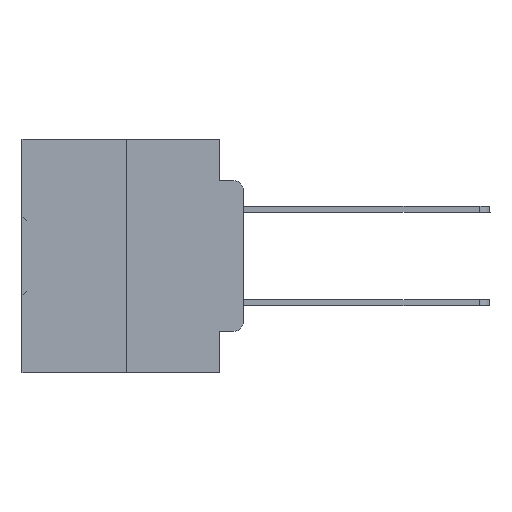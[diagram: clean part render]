
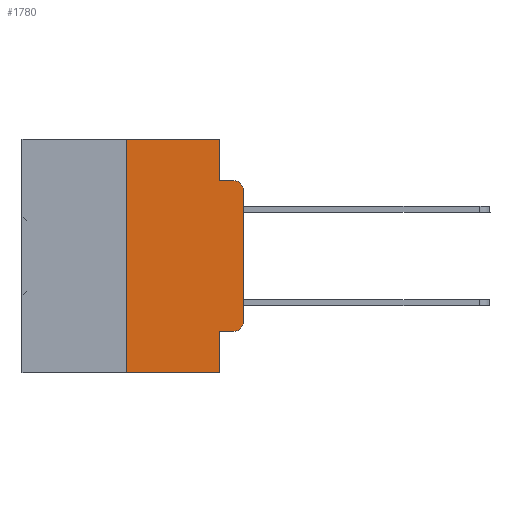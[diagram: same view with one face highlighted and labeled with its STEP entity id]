
A CAD part, left-side view. The second image highlights one B-rep face of the part: STEP entity #1780.
In plain terms, the highlighted planar face has unit normal (-1, 0, 0).
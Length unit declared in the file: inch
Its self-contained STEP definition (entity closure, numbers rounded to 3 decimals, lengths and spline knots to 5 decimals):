
#184 = ORIENTED_EDGE ( 'NONE', *, *, #28076, .T. ) ;
#339 = DIRECTION ( 'NONE',  ( -1., 0., 0. ) ) ;
#488 = LINE ( 'NONE', #30075, #31539 ) ;
#667 = DIRECTION ( 'NONE',  ( 0., -1., 0. ) ) ;
#1204 = CIRCLE ( 'NONE', #9389, 0.02 ) ;
#1375 = CARTESIAN_POINT ( 'NONE',  ( 0., 0.02, -0.1085 ) ) ;
#1562 = ORIENTED_EDGE ( 'NONE', *, *, #8006, .T. ) ;
#1780 = ADVANCED_FACE ( 'NONE', ( #26028 ), #14416, .F. ) ;
#1823 = CARTESIAN_POINT ( 'NONE',  ( 0., 0.051, 0. ) ) ;
#2549 = AXIS2_PLACEMENT_3D ( 'NONE', #1375, #21821, #4304 ) ;
#2571 = VECTOR ( 'NONE', #5016, 39.37008 ) ;
#3223 = EDGE_LOOP ( 'NONE', ( #20301, #1562, #24870, #10236, #19879, #22594, #184, #31233, #27148, #28967 ) ) ;
#3599 = CARTESIAN_POINT ( 'NONE',  ( 0., 0.051, 0. ) ) ;
#3652 = DIRECTION ( 'NONE',  ( 0., -1., 0. ) ) ;
#3897 = CARTESIAN_POINT ( 'NONE',  ( 0., 0.02, -0.0885 ) ) ;
#4127 = EDGE_CURVE ( 'NONE', #21525, #31232, #7282, .T. ) ;
#4304 = DIRECTION ( 'NONE',  ( 0., 0., -1. ) ) ;
#4619 = CARTESIAN_POINT ( 'NONE',  ( 0., 0.25, 0. ) ) ;
#5016 = DIRECTION ( 'NONE',  ( 0., -1., 0. ) ) ;
#5712 = VERTEX_POINT ( 'NONE', #8740 ) ;
#6056 = EDGE_CURVE ( 'NONE', #31232, #13509, #18146, .T. ) ;
#6818 = LINE ( 'NONE', #22904, #36858 ) ;
#6942 = DIRECTION ( 'NONE',  ( 1., 0., 0. ) ) ;
#7282 = LINE ( 'NONE', #3599, #21940 ) ;
#7541 = CARTESIAN_POINT ( 'NONE',  ( 0., 0.051, 0. ) ) ;
#7807 = CARTESIAN_POINT ( 'NONE',  ( 0., 0.051, -0.0885 ) ) ;
#8006 = EDGE_CURVE ( 'NONE', #28084, #13509, #13012, .T. ) ;
#8740 = CARTESIAN_POINT ( 'NONE',  ( 0., 0.051, -0.4115 ) ) ;
#8937 = VERTEX_POINT ( 'NONE', #34529 ) ;
#9389 = AXIS2_PLACEMENT_3D ( 'NONE', #17890, #339, #20785 ) ;
#10236 = ORIENTED_EDGE ( 'NONE', *, *, #4127, .F. ) ;
#10622 = VERTEX_POINT ( 'NONE', #4619 ) ;
#10963 = DIRECTION ( 'NONE',  ( 0., -1., 0. ) ) ;
#10972 = VECTOR ( 'NONE', #667, 39.37008 ) ;
#12506 = DIRECTION ( 'NONE',  ( 0., 0., 1. ) ) ;
#13012 = CIRCLE ( 'NONE', #2549, 0.02 ) ;
#13450 = DIRECTION ( 'NONE',  ( 0., 0., -1. ) ) ;
#13509 = VERTEX_POINT ( 'NONE', #3897 ) ;
#14416 = PLANE ( 'NONE',  #29544 ) ;
#15369 = CARTESIAN_POINT ( 'NONE',  ( 0., 0., -0.1085 ) ) ;
#15442 = EDGE_CURVE ( 'NONE', #10622, #21525, #24376, .T. ) ;
#16745 = DIRECTION ( 'NONE',  ( 0., 0., -1. ) ) ;
#16824 = VERTEX_POINT ( 'NONE', #33489 ) ;
#17862 = EDGE_CURVE ( 'NONE', #16824, #28084, #488, .T. ) ;
#17890 = CARTESIAN_POINT ( 'NONE',  ( 0., 0.02, -0.3915 ) ) ;
#18146 = LINE ( 'NONE', #7807, #2571 ) ;
#18437 = LINE ( 'NONE', #1823, #20250 ) ;
#19879 = ORIENTED_EDGE ( 'NONE', *, *, #15442, .F. ) ;
#19896 = CARTESIAN_POINT ( 'NONE',  ( 0., 0.051, -0.5 ) ) ;
#20250 = VECTOR ( 'NONE', #13450, 39.37008 ) ;
#20301 = ORIENTED_EDGE ( 'NONE', *, *, #17862, .T. ) ;
#20521 = EDGE_CURVE ( 'NONE', #26332, #16824, #1204, .T. ) ;
#20785 = DIRECTION ( 'NONE',  ( 0., 0., -1. ) ) ;
#21156 = CARTESIAN_POINT ( 'NONE',  ( 0., 0.473, 0. ) ) ;
#21525 = VERTEX_POINT ( 'NONE', #7541 ) ;
#21821 = DIRECTION ( 'NONE',  ( -1., 0., 0. ) ) ;
#21940 = VECTOR ( 'NONE', #24052, 39.37008 ) ;
#22212 = LINE ( 'NONE', #37016, #30849 ) ;
#22529 = VECTOR ( 'NONE', #3652, 39.37008 ) ;
#22594 = ORIENTED_EDGE ( 'NONE', *, *, #34113, .F. ) ;
#22904 = CARTESIAN_POINT ( 'NONE',  ( 0., 0.25, 0. ) ) ;
#24052 = DIRECTION ( 'NONE',  ( 0., 0., -1. ) ) ;
#24376 = LINE ( 'NONE', #21156, #22529 ) ;
#24422 = CARTESIAN_POINT ( 'NONE',  ( 0., 0.02, -0.4115 ) ) ;
#24870 = ORIENTED_EDGE ( 'NONE', *, *, #6056, .F. ) ;
#26028 = FACE_OUTER_BOUND ( 'NONE', #3223, .T. ) ;
#26332 = VERTEX_POINT ( 'NONE', #24422 ) ;
#26478 = LINE ( 'NONE', #29753, #10972 ) ;
#27148 = ORIENTED_EDGE ( 'NONE', *, *, #30275, .T. ) ;
#27285 = VERTEX_POINT ( 'NONE', #19896 ) ;
#27552 = CARTESIAN_POINT ( 'NONE',  ( 0., 0.473, 0. ) ) ;
#28076 = EDGE_CURVE ( 'NONE', #8937, #27285, #26478, .T. ) ;
#28084 = VERTEX_POINT ( 'NONE', #15369 ) ;
#28967 = ORIENTED_EDGE ( 'NONE', *, *, #20521, .T. ) ;
#29544 = AXIS2_PLACEMENT_3D ( 'NONE', #27552, #6942, #16745 ) ;
#29753 = CARTESIAN_POINT ( 'NONE',  ( 0., 0.473, -0.5 ) ) ;
#30075 = CARTESIAN_POINT ( 'NONE',  ( 0., 0., 0. ) ) ;
#30275 = EDGE_CURVE ( 'NONE', #5712, #26332, #22212, .T. ) ;
#30849 = VECTOR ( 'NONE', #10963, 39.37008 ) ;
#31232 = VERTEX_POINT ( 'NONE', #35562 ) ;
#31233 = ORIENTED_EDGE ( 'NONE', *, *, #32190, .F. ) ;
#31539 = VECTOR ( 'NONE', #12506, 39.37008 ) ;
#31664 = DIRECTION ( 'NONE',  ( 0., 0., 1. ) ) ;
#32190 = EDGE_CURVE ( 'NONE', #5712, #27285, #18437, .T. ) ;
#33489 = CARTESIAN_POINT ( 'NONE',  ( 0., 0., -0.3915 ) ) ;
#34113 = EDGE_CURVE ( 'NONE', #8937, #10622, #6818, .T. ) ;
#34529 = CARTESIAN_POINT ( 'NONE',  ( 0., 0.25, -0.5 ) ) ;
#35562 = CARTESIAN_POINT ( 'NONE',  ( 0., 0.051, -0.0885 ) ) ;
#36858 = VECTOR ( 'NONE', #31664, 39.37008 ) ;
#37016 = CARTESIAN_POINT ( 'NONE',  ( 0., 0.051, -0.4115 ) ) ;
